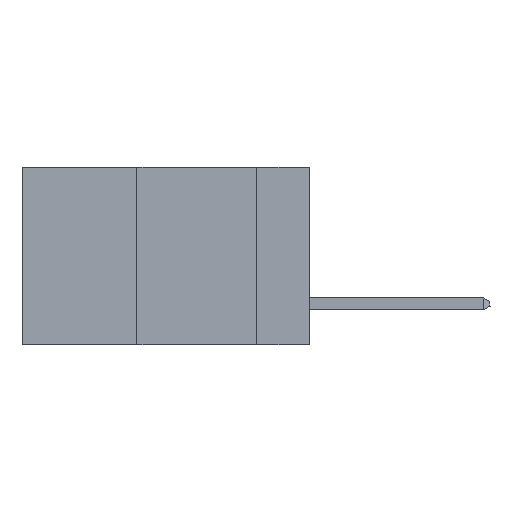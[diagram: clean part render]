
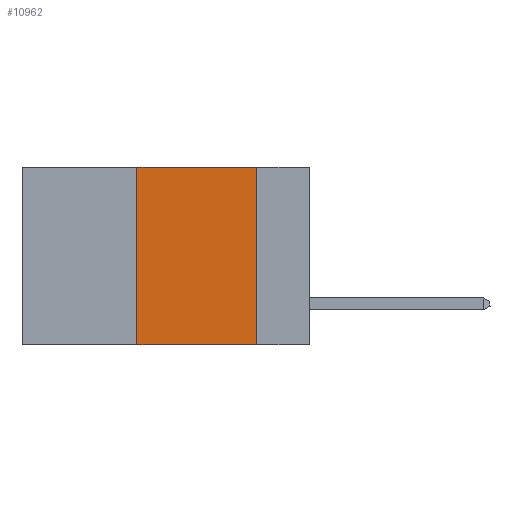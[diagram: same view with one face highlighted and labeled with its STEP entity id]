
A CAD part, left-side view. The second image highlights one B-rep face of the part: STEP entity #10962.
In plain terms, the highlighted planar face has unit normal (-1, 0, 0).
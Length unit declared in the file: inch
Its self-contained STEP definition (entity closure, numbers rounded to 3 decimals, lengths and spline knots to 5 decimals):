
#104 = CARTESIAN_POINT ( 'NONE',  ( 0., 0.36, 0. ) ) ;
#327 = ORIENTED_EDGE ( 'NONE', *, *, #5111, .F. ) ;
#1015 = PLANE ( 'NONE',  #10919 ) ;
#1783 = CARTESIAN_POINT ( 'NONE',  ( 0., 0.11, 0. ) ) ;
#2014 = VERTEX_POINT ( 'NONE', #11430 ) ;
#2069 = DIRECTION ( 'NONE',  ( 1., 0., 0. ) ) ;
#2873 = DIRECTION ( 'NONE',  ( 0., 0., 1. ) ) ;
#2887 = DIRECTION ( 'NONE',  ( 0., 0., -1. ) ) ;
#2961 = ORIENTED_EDGE ( 'NONE', *, *, #5303, .T. ) ;
#4069 = CARTESIAN_POINT ( 'NONE',  ( 0., 0.36, 0. ) ) ;
#4245 = FACE_OUTER_BOUND ( 'NONE', #5213, .T. ) ;
#4436 = ORIENTED_EDGE ( 'NONE', *, *, #14034, .F. ) ;
#4453 = VERTEX_POINT ( 'NONE', #7228 ) ;
#5111 = EDGE_CURVE ( 'NONE', #4453, #8210, #12151, .T. ) ;
#5150 = CARTESIAN_POINT ( 'NONE',  ( 0., 0.11, 0. ) ) ;
#5213 = EDGE_LOOP ( 'NONE', ( #11627, #4436, #327, #2961 ) ) ;
#5303 = EDGE_CURVE ( 'NONE', #4453, #2014, #12142, .T. ) ;
#5446 = VECTOR ( 'NONE', #8709, 39.37008 ) ;
#5735 = EDGE_CURVE ( 'NONE', #7533, #2014, #12972, .T. ) ;
#6155 = VECTOR ( 'NONE', #2873, 39.37008 ) ;
#6425 = DIRECTION ( 'NONE',  ( 0., -1., 0. ) ) ;
#7167 = VECTOR ( 'NONE', #2887, 39.37008 ) ;
#7228 = CARTESIAN_POINT ( 'NONE',  ( 0., 0.36, -0.37 ) ) ;
#7533 = VERTEX_POINT ( 'NONE', #1783 ) ;
#8210 = VERTEX_POINT ( 'NONE', #104 ) ;
#8709 = DIRECTION ( 'NONE',  ( 0., -1., 0. ) ) ;
#8918 = DIRECTION ( 'NONE',  ( 0., 0., -1. ) ) ;
#10823 = LINE ( 'NONE', #14265, #14108 ) ;
#10919 = AXIS2_PLACEMENT_3D ( 'NONE', #11058, #2069, #8918 ) ;
#10962 = ADVANCED_FACE ( 'NONE', ( #4245 ), #1015, .F. ) ;
#11058 = CARTESIAN_POINT ( 'NONE',  ( 0., 0.6, 0. ) ) ;
#11132 = CARTESIAN_POINT ( 'NONE',  ( 0., 0.6, -0.37 ) ) ;
#11430 = CARTESIAN_POINT ( 'NONE',  ( 0., 0.11, -0.37 ) ) ;
#11627 = ORIENTED_EDGE ( 'NONE', *, *, #5735, .F. ) ;
#12142 = LINE ( 'NONE', #11132, #5446 ) ;
#12151 = LINE ( 'NONE', #4069, #6155 ) ;
#12972 = LINE ( 'NONE', #5150, #7167 ) ;
#14034 = EDGE_CURVE ( 'NONE', #8210, #7533, #10823, .T. ) ;
#14108 = VECTOR ( 'NONE', #6425, 39.37008 ) ;
#14265 = CARTESIAN_POINT ( 'NONE',  ( 0., 0.6, 0. ) ) ;
